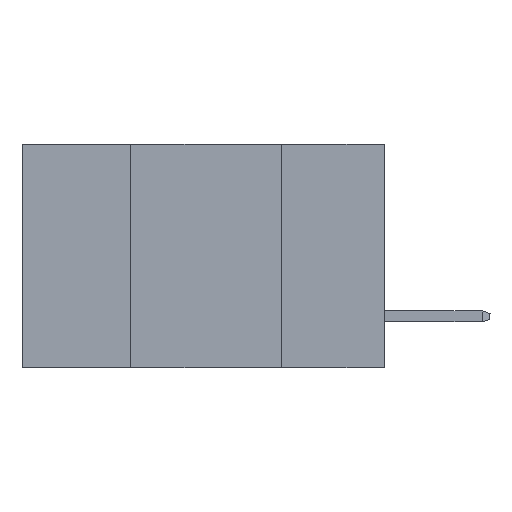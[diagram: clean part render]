
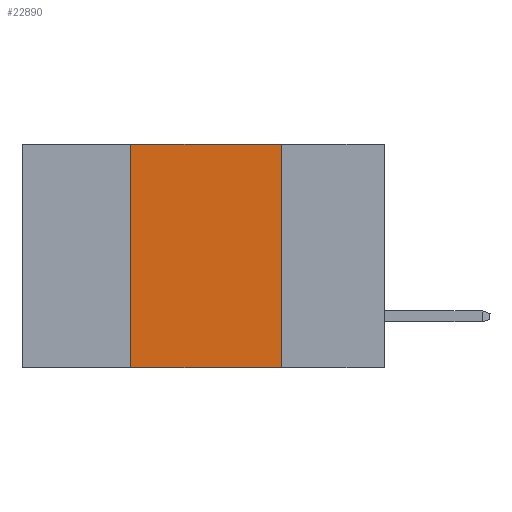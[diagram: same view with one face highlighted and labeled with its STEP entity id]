
A CAD part, left-side view. The second image highlights one B-rep face of the part: STEP entity #22890.
In plain terms, the highlighted planar face has unit normal (-1, 0, 0).
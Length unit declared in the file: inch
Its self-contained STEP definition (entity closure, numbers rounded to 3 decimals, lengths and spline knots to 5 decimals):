
#114 = EDGE_CURVE ( 'NONE', #21349, #2525, #22690, .T. ) ;
#123 = LINE ( 'NONE', #3618, #3516 ) ;
#910 = CARTESIAN_POINT ( 'NONE',  ( 0., 0.17, 0. ) ) ;
#1971 = VERTEX_POINT ( 'NONE', #20919 ) ;
#2466 = ORIENTED_EDGE ( 'NONE', *, *, #114, .T. ) ;
#2525 = VERTEX_POINT ( 'NONE', #18090 ) ;
#3053 = ORIENTED_EDGE ( 'NONE', *, *, #21362, .F. ) ;
#3516 = VECTOR ( 'NONE', #9325, 39.37008 ) ;
#3618 = CARTESIAN_POINT ( 'NONE',  ( 0., 0.17, -0.37 ) ) ;
#4652 = PLANE ( 'NONE',  #7224 ) ;
#7224 = AXIS2_PLACEMENT_3D ( 'NONE', #11763, #9667, #18853 ) ;
#9325 = DIRECTION ( 'NONE',  ( 0., 0., -1. ) ) ;
#9667 = DIRECTION ( 'NONE',  ( 1., 0., 0. ) ) ;
#9940 = VECTOR ( 'NONE', #12111, 39.37008 ) ;
#10270 = CARTESIAN_POINT ( 'NONE',  ( 0., 0.6, 0. ) ) ;
#11763 = CARTESIAN_POINT ( 'NONE',  ( 0., 0.6, 0. ) ) ;
#12014 = CARTESIAN_POINT ( 'NONE',  ( 0., 0.42, -0.37 ) ) ;
#12111 = DIRECTION ( 'NONE',  ( 0., -1., 0. ) ) ;
#12781 = EDGE_CURVE ( 'NONE', #21349, #1971, #20663, .T. ) ;
#15361 = ORIENTED_EDGE ( 'NONE', *, *, #21422, .F. ) ;
#15662 = DIRECTION ( 'NONE',  ( 0., 0., 1. ) ) ;
#16658 = VERTEX_POINT ( 'NONE', #910 ) ;
#17100 = FACE_OUTER_BOUND ( 'NONE', #18244, .T. ) ;
#17278 = VECTOR ( 'NONE', #22715, 39.37008 ) ;
#17400 = CARTESIAN_POINT ( 'NONE',  ( 0., 0.42, -0.37 ) ) ;
#18090 = CARTESIAN_POINT ( 'NONE',  ( 0., 0.17, -0.37 ) ) ;
#18244 = EDGE_LOOP ( 'NONE', ( #15361, #3053, #21252, #2466 ) ) ;
#18853 = DIRECTION ( 'NONE',  ( 0., 0., -1. ) ) ;
#19117 = LINE ( 'NONE', #10270, #17278 ) ;
#19668 = CARTESIAN_POINT ( 'NONE',  ( 0., 0.6, -0.37 ) ) ;
#20663 = LINE ( 'NONE', #17400, #21312 ) ;
#20919 = CARTESIAN_POINT ( 'NONE',  ( 0., 0.42, 0. ) ) ;
#21252 = ORIENTED_EDGE ( 'NONE', *, *, #12781, .F. ) ;
#21312 = VECTOR ( 'NONE', #15662, 39.37008 ) ;
#21349 = VERTEX_POINT ( 'NONE', #12014 ) ;
#21362 = EDGE_CURVE ( 'NONE', #1971, #16658, #19117, .T. ) ;
#21422 = EDGE_CURVE ( 'NONE', #16658, #2525, #123, .T. ) ;
#22690 = LINE ( 'NONE', #19668, #9940 ) ;
#22715 = DIRECTION ( 'NONE',  ( 0., -1., 0. ) ) ;
#22890 = ADVANCED_FACE ( 'NONE', ( #17100 ), #4652, .F. ) ;
